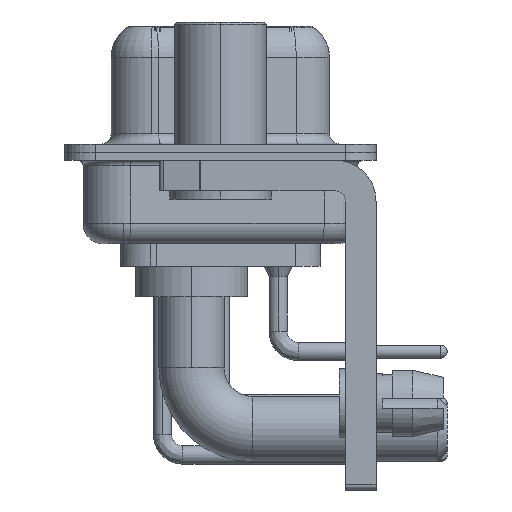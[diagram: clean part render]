
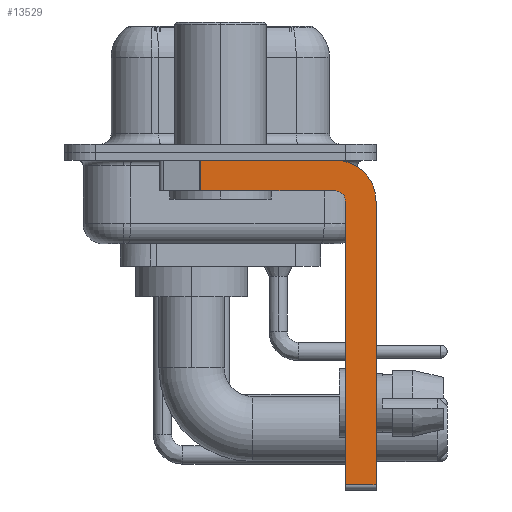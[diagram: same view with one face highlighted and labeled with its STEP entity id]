
A CAD part, left-side view. The second image highlights one B-rep face of the part: STEP entity #13529.
In plain terms, the highlighted planar face has unit normal (-1, 0, 0).
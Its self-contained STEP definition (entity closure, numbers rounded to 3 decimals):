
#75 = DIRECTION ( 'NONE',  ( 0., 0., -1. ) ) ;
#1433 = EDGE_LOOP ( 'NONE', ( #25875, #14825, #3594, #11651, #32432, #34290, #27339, #3207 ) ) ;
#1566 = EDGE_CURVE ( 'NONE', #22974, #7929, #32264, .T. ) ;
#1621 = VERTEX_POINT ( 'NONE', #2147 ) ;
#1673 = CIRCLE ( 'NONE', #7538, 2. ) ;
#2147 = CARTESIAN_POINT ( 'NONE',  ( -2.9, 0.978, -1.9 ) ) ;
#2881 = DIRECTION ( 'NONE',  ( 0., 0., -1. ) ) ;
#3032 = CARTESIAN_POINT ( 'NONE',  ( -2.9, -5.65, -1.9 ) ) ;
#3207 = ORIENTED_EDGE ( 'NONE', *, *, #21088, .F. ) ;
#3594 = ORIENTED_EDGE ( 'NONE', *, *, #24557, .F. ) ;
#6681 = AXIS2_PLACEMENT_3D ( 'NONE', #30349, #35985, #21593 ) ;
#7015 = DIRECTION ( 'NONE',  ( 0., 0., 1. ) ) ;
#7278 = CARTESIAN_POINT ( 'NONE',  ( -2.9, -6.15, -16.35 ) ) ;
#7468 = CARTESIAN_POINT ( 'NONE',  ( -2.9, -5.65, -1.9 ) ) ;
#7538 = AXIS2_PLACEMENT_3D ( 'NONE', #27839, #13990, #75 ) ;
#7929 = VERTEX_POINT ( 'NONE', #14178 ) ;
#8056 = DIRECTION ( 'NONE',  ( -1., 0., 0. ) ) ;
#8365 = LINE ( 'NONE', #17477, #10926 ) ;
#9415 = VECTOR ( 'NONE', #19996, 1000. ) ;
#9482 = VECTOR ( 'NONE', #29431, 1000. ) ;
#10779 = CARTESIAN_POINT ( 'NONE',  ( -2.9, -5.65, -2.4 ) ) ;
#10926 = VECTOR ( 'NONE', #2881, 1000. ) ;
#11651 = ORIENTED_EDGE ( 'NONE', *, *, #30794, .F. ) ;
#12321 = CARTESIAN_POINT ( 'NONE',  ( -2.9, -6.15, -16.6 ) ) ;
#12959 = CARTESIAN_POINT ( 'NONE',  ( -2.9, -5.65, -0.4 ) ) ;
#13415 = PLANE ( 'NONE',  #6681 ) ;
#13529 = ADVANCED_FACE ( 'NONE', ( #16310 ), #13415, .F. ) ;
#13990 = DIRECTION ( 'NONE',  ( 1., 0., 0. ) ) ;
#14178 = CARTESIAN_POINT ( 'NONE',  ( -2.9, -7.65, -16.35 ) ) ;
#14825 = ORIENTED_EDGE ( 'NONE', *, *, #16005, .T. ) ;
#15564 = VERTEX_POINT ( 'NONE', #19878 ) ;
#16005 = EDGE_CURVE ( 'NONE', #23481, #1621, #8365, .T. ) ;
#16122 = CARTESIAN_POINT ( 'NONE',  ( -2.9, -7.65, -2.4 ) ) ;
#16310 = FACE_OUTER_BOUND ( 'NONE', #1433, .T. ) ;
#17477 = CARTESIAN_POINT ( 'NONE',  ( -2.9, 0.978, -1.9 ) ) ;
#17842 = VECTOR ( 'NONE', #21520, 1000. ) ;
#17886 = VECTOR ( 'NONE', #7015, 1000. ) ;
#18284 = CARTESIAN_POINT ( 'NONE',  ( -2.9, -7.65, -2.4 ) ) ;
#19398 = EDGE_CURVE ( 'NONE', #22974, #15564, #29283, .T. ) ;
#19878 = CARTESIAN_POINT ( 'NONE',  ( -2.9, -6.15, -2.4 ) ) ;
#19996 = DIRECTION ( 'NONE',  ( 0., 1., 0. ) ) ;
#20650 = LINE ( 'NONE', #18284, #9482 ) ;
#21088 = EDGE_CURVE ( 'NONE', #25596, #34310, #1673, .T. ) ;
#21520 = DIRECTION ( 'NONE',  ( 0., -1., 0. ) ) ;
#21593 = DIRECTION ( 'NONE',  ( 0., 0., -1. ) ) ;
#21678 = DIRECTION ( 'NONE',  ( 0., -1., 0. ) ) ;
#22974 = VERTEX_POINT ( 'NONE', #7278 ) ;
#23481 = VERTEX_POINT ( 'NONE', #30344 ) ;
#24557 = EDGE_CURVE ( 'NONE', #35238, #1621, #34036, .T. ) ;
#25596 = VERTEX_POINT ( 'NONE', #12959 ) ;
#25863 = AXIS2_PLACEMENT_3D ( 'NONE', #10779, #8056, #33377 ) ;
#25875 = ORIENTED_EDGE ( 'NONE', *, *, #32631, .F. ) ;
#27339 = ORIENTED_EDGE ( 'NONE', *, *, #28290, .F. ) ;
#27529 = CARTESIAN_POINT ( 'NONE',  ( -2.9, -5.65, -16.35 ) ) ;
#27839 = CARTESIAN_POINT ( 'NONE',  ( -2.9, -5.65, -2.4 ) ) ;
#28290 = EDGE_CURVE ( 'NONE', #34310, #7929, #20650, .T. ) ;
#29283 = LINE ( 'NONE', #12321, #17886 ) ;
#29431 = DIRECTION ( 'NONE',  ( 0., 0., -1. ) ) ;
#30100 = LINE ( 'NONE', #30449, #17842 ) ;
#30344 = CARTESIAN_POINT ( 'NONE',  ( -2.9, 0.978, -0.4 ) ) ;
#30349 = CARTESIAN_POINT ( 'NONE',  ( -2.9, -5.65, -2.4 ) ) ;
#30449 = CARTESIAN_POINT ( 'NONE',  ( -2.9, 3., -0.4 ) ) ;
#30649 = VECTOR ( 'NONE', #21678, 1000. ) ;
#30794 = EDGE_CURVE ( 'NONE', #15564, #35238, #31098, .T. ) ;
#31098 = CIRCLE ( 'NONE', #25863, 0.5 ) ;
#32264 = LINE ( 'NONE', #27529, #30649 ) ;
#32432 = ORIENTED_EDGE ( 'NONE', *, *, #19398, .F. ) ;
#32631 = EDGE_CURVE ( 'NONE', #23481, #25596, #30100, .T. ) ;
#33377 = DIRECTION ( 'NONE',  ( 0., 0., 1. ) ) ;
#34036 = LINE ( 'NONE', #3032, #9415 ) ;
#34290 = ORIENTED_EDGE ( 'NONE', *, *, #1566, .T. ) ;
#34310 = VERTEX_POINT ( 'NONE', #16122 ) ;
#35238 = VERTEX_POINT ( 'NONE', #7468 ) ;
#35985 = DIRECTION ( 'NONE',  ( 1., 0., 0. ) ) ;
